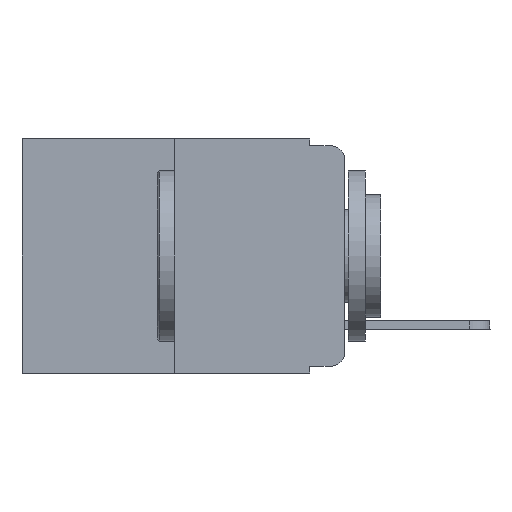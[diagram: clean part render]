
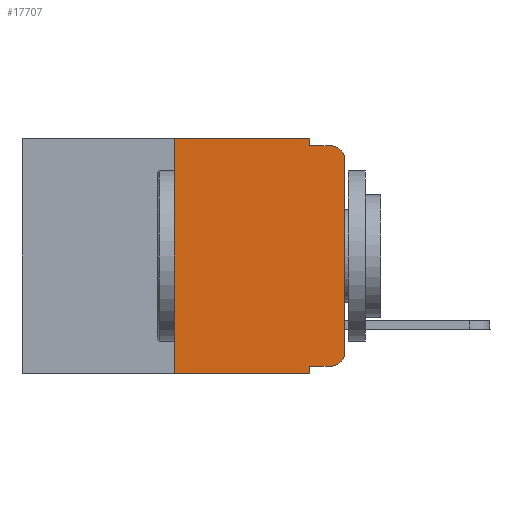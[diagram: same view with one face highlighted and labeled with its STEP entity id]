
A CAD part, left-side view. The second image highlights one B-rep face of the part: STEP entity #17707.
In plain terms, the highlighted planar face has unit normal (-1, 0, 0).
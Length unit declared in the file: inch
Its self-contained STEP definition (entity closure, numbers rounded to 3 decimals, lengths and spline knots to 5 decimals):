
#67 = CARTESIAN_POINT ( 'NONE',  ( 0., 0.473, -0.343 ) ) ;
#478 = VECTOR ( 'NONE', #3699, 39.37008 ) ;
#778 = VERTEX_POINT ( 'NONE', #18691 ) ;
#1240 = CARTESIAN_POINT ( 'NONE',  ( 0., 0.25, 0. ) ) ;
#1311 = VECTOR ( 'NONE', #3304, 39.37008 ) ;
#1610 = CARTESIAN_POINT ( 'NONE',  ( 0., 0.02, -0.01 ) ) ;
#2308 = VECTOR ( 'NONE', #7573, 39.37008 ) ;
#3304 = DIRECTION ( 'NONE',  ( 0., -1., 0. ) ) ;
#3699 = DIRECTION ( 'NONE',  ( 0., -1., 0. ) ) ;
#3938 = DIRECTION ( 'NONE',  ( -1., 0., 0. ) ) ;
#4059 = VECTOR ( 'NONE', #20018, 39.37008 ) ;
#4214 = EDGE_CURVE ( 'NONE', #20180, #18684, #17880, .T. ) ;
#4478 = CARTESIAN_POINT ( 'NONE',  ( 0., 0.051, -0.343 ) ) ;
#4845 = DIRECTION ( 'NONE',  ( 0., -1., 0. ) ) ;
#4860 = AXIS2_PLACEMENT_3D ( 'NONE', #16250, #14542, #8878 ) ;
#5239 = DIRECTION ( 'NONE',  ( -1., 0., 0. ) ) ;
#5323 = LINE ( 'NONE', #7021, #11536 ) ;
#5474 = ORIENTED_EDGE ( 'NONE', *, *, #16947, .T. ) ;
#5648 = EDGE_LOOP ( 'NONE', ( #5474, #12514, #20432, #22452, #8895, #15781, #13175, #7591, #15094, #8675 ) ) ;
#5932 = EDGE_CURVE ( 'NONE', #16940, #18840, #16954, .T. ) ;
#6198 = CARTESIAN_POINT ( 'NONE',  ( 0., 0., 0. ) ) ;
#6257 = LINE ( 'NONE', #1240, #15859 ) ;
#6297 = EDGE_CURVE ( 'NONE', #8225, #8331, #5323, .T. ) ;
#6469 = CARTESIAN_POINT ( 'NONE',  ( 0., 0.051, 0. ) ) ;
#6556 = VERTEX_POINT ( 'NONE', #16239 ) ;
#7021 = CARTESIAN_POINT ( 'NONE',  ( 0., 0.051, 0. ) ) ;
#7029 = CARTESIAN_POINT ( 'NONE',  ( 0., 0.051, -0.01 ) ) ;
#7133 = AXIS2_PLACEMENT_3D ( 'NONE', #20810, #5239, #17633 ) ;
#7476 = CIRCLE ( 'NONE', #15101, 0.02 ) ;
#7573 = DIRECTION ( 'NONE',  ( 0., 0., 1. ) ) ;
#7591 = ORIENTED_EDGE ( 'NONE', *, *, #4214, .F. ) ;
#7799 = VERTEX_POINT ( 'NONE', #12103 ) ;
#8225 = VERTEX_POINT ( 'NONE', #6469 ) ;
#8331 = VERTEX_POINT ( 'NONE', #7029 ) ;
#8675 = ORIENTED_EDGE ( 'NONE', *, *, #10069, .T. ) ;
#8765 = CARTESIAN_POINT ( 'NONE',  ( 0., 0.051, -0.01 ) ) ;
#8878 = DIRECTION ( 'NONE',  ( 0., 0., -1. ) ) ;
#8895 = ORIENTED_EDGE ( 'NONE', *, *, #18508, .F. ) ;
#8932 = CARTESIAN_POINT ( 'NONE',  ( 0., 0.473, 0. ) ) ;
#10069 = EDGE_CURVE ( 'NONE', #22223, #778, #7476, .T. ) ;
#10464 = EDGE_CURVE ( 'NONE', #20180, #22223, #19156, .T. ) ;
#10984 = CARTESIAN_POINT ( 'NONE',  ( 0., 0.02, -0.313 ) ) ;
#11536 = VECTOR ( 'NONE', #12490, 39.37008 ) ;
#11847 = VECTOR ( 'NONE', #12336, 39.37008 ) ;
#12103 = CARTESIAN_POINT ( 'NONE',  ( 0., 0.25, 0. ) ) ;
#12336 = DIRECTION ( 'NONE',  ( 0., -1., 0. ) ) ;
#12490 = DIRECTION ( 'NONE',  ( 0., 0., -1. ) ) ;
#12514 = ORIENTED_EDGE ( 'NONE', *, *, #5932, .T. ) ;
#12645 = CARTESIAN_POINT ( 'NONE',  ( 0., 0.051, 0. ) ) ;
#13175 = ORIENTED_EDGE ( 'NONE', *, *, #14480, .T. ) ;
#14176 = DIRECTION ( 'NONE',  ( 0., 0., -1. ) ) ;
#14480 = EDGE_CURVE ( 'NONE', #6556, #18684, #15539, .T. ) ;
#14542 = DIRECTION ( 'NONE',  ( 1., 0., 0. ) ) ;
#14657 = CARTESIAN_POINT ( 'NONE',  ( 0., 0.02, -0.333 ) ) ;
#14853 = CARTESIAN_POINT ( 'NONE',  ( 0., 0., -0.03 ) ) ;
#15094 = ORIENTED_EDGE ( 'NONE', *, *, #10464, .T. ) ;
#15101 = AXIS2_PLACEMENT_3D ( 'NONE', #10984, #3938, #14176 ) ;
#15121 = DIRECTION ( 'NONE',  ( 0., 0., 1. ) ) ;
#15539 = LINE ( 'NONE', #67, #20345 ) ;
#15781 = ORIENTED_EDGE ( 'NONE', *, *, #21911, .F. ) ;
#15859 = VECTOR ( 'NONE', #15121, 39.37008 ) ;
#16239 = CARTESIAN_POINT ( 'NONE',  ( 0., 0.25, -0.343 ) ) ;
#16250 = CARTESIAN_POINT ( 'NONE',  ( 0., 0.473, 0. ) ) ;
#16940 = VERTEX_POINT ( 'NONE', #14853 ) ;
#16947 = EDGE_CURVE ( 'NONE', #778, #16940, #21770, .T. ) ;
#16954 = CIRCLE ( 'NONE', #7133, 0.02 ) ;
#17464 = LINE ( 'NONE', #8932, #478 ) ;
#17633 = DIRECTION ( 'NONE',  ( 0., 0., -1. ) ) ;
#17707 = ADVANCED_FACE ( 'NONE', ( #21461 ), #19761, .F. ) ;
#17880 = LINE ( 'NONE', #12645, #4059 ) ;
#18508 = EDGE_CURVE ( 'NONE', #7799, #8225, #17464, .T. ) ;
#18684 = VERTEX_POINT ( 'NONE', #4478 ) ;
#18691 = CARTESIAN_POINT ( 'NONE',  ( 0., 0., -0.313 ) ) ;
#18840 = VERTEX_POINT ( 'NONE', #1610 ) ;
#19156 = LINE ( 'NONE', #20855, #11847 ) ;
#19761 = PLANE ( 'NONE',  #4860 ) ;
#20018 = DIRECTION ( 'NONE',  ( 0., 0., -1. ) ) ;
#20026 = CARTESIAN_POINT ( 'NONE',  ( 0., 0.051, -0.333 ) ) ;
#20180 = VERTEX_POINT ( 'NONE', #20026 ) ;
#20345 = VECTOR ( 'NONE', #4845, 39.37008 ) ;
#20432 = ORIENTED_EDGE ( 'NONE', *, *, #22029, .F. ) ;
#20564 = LINE ( 'NONE', #8765, #1311 ) ;
#20810 = CARTESIAN_POINT ( 'NONE',  ( 0., 0.02, -0.03 ) ) ;
#20855 = CARTESIAN_POINT ( 'NONE',  ( 0., 0.051, -0.333 ) ) ;
#21461 = FACE_OUTER_BOUND ( 'NONE', #5648, .T. ) ;
#21770 = LINE ( 'NONE', #6198, #2308 ) ;
#21911 = EDGE_CURVE ( 'NONE', #6556, #7799, #6257, .T. ) ;
#22029 = EDGE_CURVE ( 'NONE', #8331, #18840, #20564, .T. ) ;
#22223 = VERTEX_POINT ( 'NONE', #14657 ) ;
#22452 = ORIENTED_EDGE ( 'NONE', *, *, #6297, .F. ) ;
